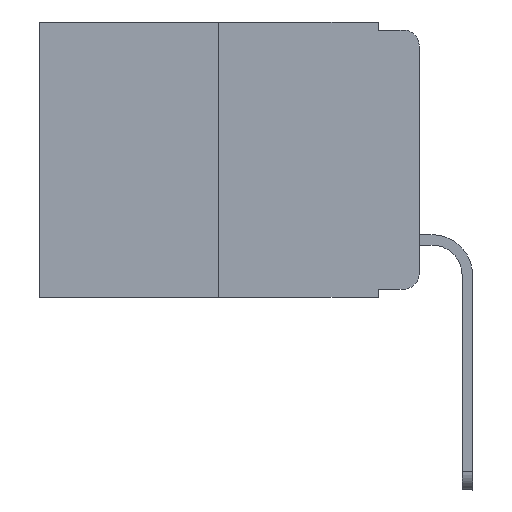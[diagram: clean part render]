
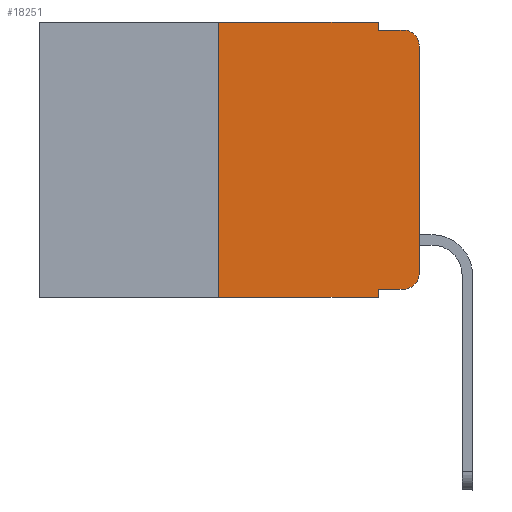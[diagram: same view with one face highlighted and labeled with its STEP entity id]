
A CAD part, left-side view. The second image highlights one B-rep face of the part: STEP entity #18251.
In plain terms, the highlighted planar face has unit normal (-1, 0, 0).
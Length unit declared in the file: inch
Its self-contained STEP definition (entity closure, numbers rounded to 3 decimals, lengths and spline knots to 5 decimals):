
#58 = CARTESIAN_POINT ( 'NONE',  ( 0., 0.02, -0.333 ) ) ;
#544 = VECTOR ( 'NONE', #15409, 39.37008 ) ;
#745 = DIRECTION ( 'NONE',  ( 0., 0., 1. ) ) ;
#973 = LINE ( 'NONE', #3960, #9937 ) ;
#1163 = DIRECTION ( 'NONE',  ( -1., 0., 0. ) ) ;
#1546 = VERTEX_POINT ( 'NONE', #8903 ) ;
#1547 = ORIENTED_EDGE ( 'NONE', *, *, #9585, .T. ) ;
#1609 = CARTESIAN_POINT ( 'NONE',  ( 0., 0.473, -0.343 ) ) ;
#1796 = DIRECTION ( 'NONE',  ( 0., -1., 0. ) ) ;
#1988 = CARTESIAN_POINT ( 'NONE',  ( 0., 0.02, -0.01 ) ) ;
#2202 = CIRCLE ( 'NONE', #9129, 0.02 ) ;
#2436 = CARTESIAN_POINT ( 'NONE',  ( 0., 0., -0.313 ) ) ;
#2472 = EDGE_CURVE ( 'NONE', #13547, #11216, #17962, .T. ) ;
#2500 = CARTESIAN_POINT ( 'NONE',  ( 0., 0.02, -0.03 ) ) ;
#2529 = ORIENTED_EDGE ( 'NONE', *, *, #7569, .F. ) ;
#2545 = VECTOR ( 'NONE', #11283, 39.37008 ) ;
#2689 = DIRECTION ( 'NONE',  ( 0., 0., -1. ) ) ;
#3136 = FACE_OUTER_BOUND ( 'NONE', #17458, .T. ) ;
#3175 = EDGE_CURVE ( 'NONE', #1546, #19319, #12438, .T. ) ;
#3458 = CARTESIAN_POINT ( 'NONE',  ( 0., 0.051, 0. ) ) ;
#3554 = LINE ( 'NONE', #3458, #2545 ) ;
#3679 = CARTESIAN_POINT ( 'NONE',  ( 0., 0., -0.03 ) ) ;
#3960 = CARTESIAN_POINT ( 'NONE',  ( 0., 0.473, 0. ) ) ;
#4036 = VECTOR ( 'NONE', #19878, 39.37008 ) ;
#4139 = CARTESIAN_POINT ( 'NONE',  ( 0., 0.25, -0.343 ) ) ;
#4420 = EDGE_CURVE ( 'NONE', #15920, #13547, #3554, .T. ) ;
#5020 = CARTESIAN_POINT ( 'NONE',  ( 0., 0.051, 0. ) ) ;
#5192 = EDGE_CURVE ( 'NONE', #17390, #11216, #8727, .T. ) ;
#6220 = DIRECTION ( 'NONE',  ( 0., 0., -1. ) ) ;
#6280 = CARTESIAN_POINT ( 'NONE',  ( 0., 0.02, -0.313 ) ) ;
#6623 = CARTESIAN_POINT ( 'NONE',  ( 0., 0.473, 0. ) ) ;
#6731 = ORIENTED_EDGE ( 'NONE', *, *, #2472, .F. ) ;
#7569 = EDGE_CURVE ( 'NONE', #18121, #15920, #973, .T. ) ;
#7729 = CARTESIAN_POINT ( 'NONE',  ( 0., 0.051, -0.343 ) ) ;
#7896 = VECTOR ( 'NONE', #1796, 39.37008 ) ;
#8048 = VERTEX_POINT ( 'NONE', #4139 ) ;
#8160 = PLANE ( 'NONE',  #15778 ) ;
#8446 = VERTEX_POINT ( 'NONE', #2436 ) ;
#8727 = CIRCLE ( 'NONE', #13346, 0.02 ) ;
#8903 = CARTESIAN_POINT ( 'NONE',  ( 0., 0.051, -0.333 ) ) ;
#9105 = CARTESIAN_POINT ( 'NONE',  ( 0., 0.25, 0. ) ) ;
#9129 = AXIS2_PLACEMENT_3D ( 'NONE', #6280, #14121, #2689 ) ;
#9303 = CARTESIAN_POINT ( 'NONE',  ( 0., 0.051, 0. ) ) ;
#9329 = CARTESIAN_POINT ( 'NONE',  ( 0., 0.051, -0.333 ) ) ;
#9372 = EDGE_CURVE ( 'NONE', #8048, #18121, #16420, .T. ) ;
#9585 = EDGE_CURVE ( 'NONE', #8446, #17390, #13561, .T. ) ;
#9785 = ORIENTED_EDGE ( 'NONE', *, *, #4420, .F. ) ;
#9937 = VECTOR ( 'NONE', #11786, 39.37008 ) ;
#9977 = EDGE_CURVE ( 'NONE', #19319, #8446, #2202, .T. ) ;
#10100 = ORIENTED_EDGE ( 'NONE', *, *, #9372, .F. ) ;
#10658 = EDGE_CURVE ( 'NONE', #8048, #13147, #14201, .T. ) ;
#10937 = ORIENTED_EDGE ( 'NONE', *, *, #5192, .T. ) ;
#11216 = VERTEX_POINT ( 'NONE', #1988 ) ;
#11283 = DIRECTION ( 'NONE',  ( 0., 0., -1. ) ) ;
#11637 = DIRECTION ( 'NONE',  ( 0., -1., 0. ) ) ;
#11763 = CARTESIAN_POINT ( 'NONE',  ( 0., 0.25, 0. ) ) ;
#11786 = DIRECTION ( 'NONE',  ( 0., -1., 0. ) ) ;
#12438 = LINE ( 'NONE', #9329, #7896 ) ;
#12644 = DIRECTION ( 'NONE',  ( 0., -1., 0. ) ) ;
#12931 = VECTOR ( 'NONE', #745, 39.37008 ) ;
#13147 = VERTEX_POINT ( 'NONE', #7729 ) ;
#13346 = AXIS2_PLACEMENT_3D ( 'NONE', #2500, #1163, #15089 ) ;
#13547 = VERTEX_POINT ( 'NONE', #20060 ) ;
#13561 = LINE ( 'NONE', #15105, #4036 ) ;
#13689 = ORIENTED_EDGE ( 'NONE', *, *, #9977, .T. ) ;
#14121 = DIRECTION ( 'NONE',  ( -1., 0., 0. ) ) ;
#14201 = LINE ( 'NONE', #1609, #14465 ) ;
#14465 = VECTOR ( 'NONE', #12644, 39.37008 ) ;
#14816 = ORIENTED_EDGE ( 'NONE', *, *, #3175, .T. ) ;
#15089 = DIRECTION ( 'NONE',  ( 0., 0., -1. ) ) ;
#15105 = CARTESIAN_POINT ( 'NONE',  ( 0., 0., 0. ) ) ;
#15409 = DIRECTION ( 'NONE',  ( 0., 0., -1. ) ) ;
#15778 = AXIS2_PLACEMENT_3D ( 'NONE', #6623, #20380, #6220 ) ;
#15920 = VERTEX_POINT ( 'NONE', #5020 ) ;
#16073 = EDGE_CURVE ( 'NONE', #1546, #13147, #20376, .T. ) ;
#16420 = LINE ( 'NONE', #11763, #12931 ) ;
#17390 = VERTEX_POINT ( 'NONE', #3679 ) ;
#17458 = EDGE_LOOP ( 'NONE', ( #1547, #10937, #6731, #9785, #2529, #10100, #20348, #19484, #14816, #13689 ) ) ;
#17962 = LINE ( 'NONE', #19407, #18819 ) ;
#18121 = VERTEX_POINT ( 'NONE', #9105 ) ;
#18251 = ADVANCED_FACE ( 'NONE', ( #3136 ), #8160, .F. ) ;
#18819 = VECTOR ( 'NONE', #11637, 39.37008 ) ;
#19319 = VERTEX_POINT ( 'NONE', #58 ) ;
#19407 = CARTESIAN_POINT ( 'NONE',  ( 0., 0.051, -0.01 ) ) ;
#19484 = ORIENTED_EDGE ( 'NONE', *, *, #16073, .F. ) ;
#19878 = DIRECTION ( 'NONE',  ( 0., 0., 1. ) ) ;
#20060 = CARTESIAN_POINT ( 'NONE',  ( 0., 0.051, -0.01 ) ) ;
#20348 = ORIENTED_EDGE ( 'NONE', *, *, #10658, .T. ) ;
#20376 = LINE ( 'NONE', #9303, #544 ) ;
#20380 = DIRECTION ( 'NONE',  ( 1., 0., 0. ) ) ;
